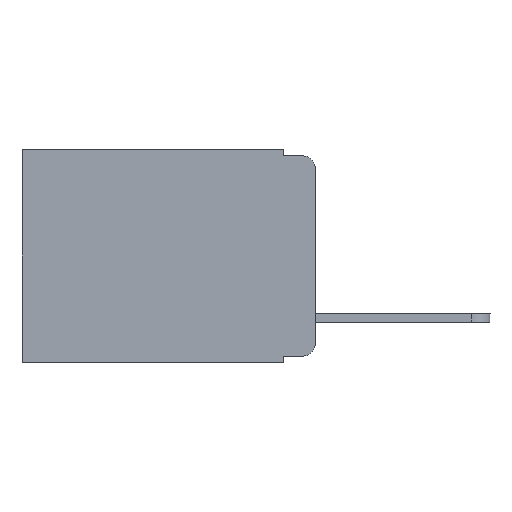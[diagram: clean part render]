
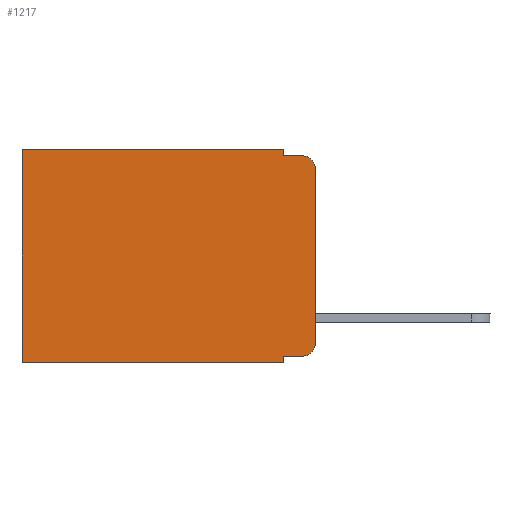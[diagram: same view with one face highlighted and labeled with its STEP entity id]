
A CAD part, left-side view. The second image highlights one B-rep face of the part: STEP entity #1217.
In plain terms, the highlighted planar face has unit normal (-1, 0, 0).
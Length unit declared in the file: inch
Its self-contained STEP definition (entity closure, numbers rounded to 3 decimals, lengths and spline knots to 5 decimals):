
#70 = LINE ( 'NONE', #7449, #6795 ) ;
#128 = DIRECTION ( 'NONE',  ( 0., -1., 0. ) ) ;
#259 = DIRECTION ( 'NONE',  ( 1., 0., 0. ) ) ;
#379 = LINE ( 'NONE', #4510, #958 ) ;
#500 = AXIS2_PLACEMENT_3D ( 'NONE', #8496, #259, #9436 ) ;
#527 = VECTOR ( 'NONE', #7770, 39.37008 ) ;
#958 = VECTOR ( 'NONE', #9495, 39.37008 ) ;
#1052 = ORIENTED_EDGE ( 'NONE', *, *, #6615, .T. ) ;
#1217 = ADVANCED_FACE ( 'NONE', ( #2091 ), #8603, .F. ) ;
#1247 = VERTEX_POINT ( 'NONE', #5398 ) ;
#1277 = EDGE_CURVE ( 'NONE', #10325, #5778, #3672, .T. ) ;
#1476 = EDGE_CURVE ( 'NONE', #10198, #7300, #3447, .T. ) ;
#2063 = EDGE_LOOP ( 'NONE', ( #9683, #9209, #2911, #2968, #3103, #5845, #3610, #7647, #1052, #7793 ) ) ;
#2086 = DIRECTION ( 'NONE',  ( 0., 0., -1. ) ) ;
#2091 = FACE_OUTER_BOUND ( 'NONE', #2063, .T. ) ;
#2202 = EDGE_CURVE ( 'NONE', #8750, #1247, #2500, .T. ) ;
#2421 = VECTOR ( 'NONE', #4393, 39.37008 ) ;
#2500 = CIRCLE ( 'NONE', #3886, 0.02 ) ;
#2911 = ORIENTED_EDGE ( 'NONE', *, *, #9700, .F. ) ;
#2965 = VERTEX_POINT ( 'NONE', #10240 ) ;
#2968 = ORIENTED_EDGE ( 'NONE', *, *, #1476, .F. ) ;
#3103 = ORIENTED_EDGE ( 'NONE', *, *, #5507, .T. ) ;
#3174 = EDGE_CURVE ( 'NONE', #8750, #7271, #70, .T. ) ;
#3294 = DIRECTION ( 'NONE',  ( 0., 0., -1. ) ) ;
#3352 = CARTESIAN_POINT ( 'NONE',  ( 0.298, 0.051, -0.343 ) ) ;
#3365 = VERTEX_POINT ( 'NONE', #7817 ) ;
#3447 = LINE ( 'NONE', #4275, #4166 ) ;
#3610 = ORIENTED_EDGE ( 'NONE', *, *, #1277, .F. ) ;
#3672 = LINE ( 'NONE', #6968, #2421 ) ;
#3679 = VECTOR ( 'NONE', #5118, 39.37008 ) ;
#3886 = AXIS2_PLACEMENT_3D ( 'NONE', #5590, #7159, #8031 ) ;
#3921 = CARTESIAN_POINT ( 'NONE',  ( 0.298, 0.051, -0.01 ) ) ;
#4166 = VECTOR ( 'NONE', #3294, 39.37008 ) ;
#4275 = CARTESIAN_POINT ( 'NONE',  ( 0.298, 0.051, 0. ) ) ;
#4365 = CARTESIAN_POINT ( 'NONE',  ( 0.298, 0.051, 0. ) ) ;
#4393 = DIRECTION ( 'NONE',  ( 0., 1., 0. ) ) ;
#4510 = CARTESIAN_POINT ( 'NONE',  ( 0.298, 0.051, -0.01 ) ) ;
#4614 = VERTEX_POINT ( 'NONE', #10211 ) ;
#5053 = EDGE_CURVE ( 'NONE', #4614, #7271, #9232, .T. ) ;
#5118 = DIRECTION ( 'NONE',  ( 0., 0., -1. ) ) ;
#5224 = LINE ( 'NONE', #6079, #527 ) ;
#5264 = EDGE_CURVE ( 'NONE', #2965, #5778, #7232, .T. ) ;
#5293 = CARTESIAN_POINT ( 'NONE',  ( 0.298, 0., -0.03 ) ) ;
#5398 = CARTESIAN_POINT ( 'NONE',  ( 0.298, 0.02, -0.01 ) ) ;
#5404 = AXIS2_PLACEMENT_3D ( 'NONE', #6912, #7785, #8599 ) ;
#5507 = EDGE_CURVE ( 'NONE', #10198, #2965, #5224, .T. ) ;
#5564 = CARTESIAN_POINT ( 'NONE',  ( 0.298, 0.051, 0. ) ) ;
#5590 = CARTESIAN_POINT ( 'NONE',  ( 0.298, 0.02, -0.03 ) ) ;
#5664 = CARTESIAN_POINT ( 'NONE',  ( 0.298, 0.051, -0.333 ) ) ;
#5778 = VERTEX_POINT ( 'NONE', #9292 ) ;
#5845 = ORIENTED_EDGE ( 'NONE', *, *, #5264, .T. ) ;
#6079 = CARTESIAN_POINT ( 'NONE',  ( 0.298, 0., 0. ) ) ;
#6615 = EDGE_CURVE ( 'NONE', #3365, #4614, #6744, .T. ) ;
#6744 = LINE ( 'NONE', #5664, #9224 ) ;
#6795 = VECTOR ( 'NONE', #7395, 39.37008 ) ;
#6912 = CARTESIAN_POINT ( 'NONE',  ( 0.298, 0.02, -0.313 ) ) ;
#6968 = CARTESIAN_POINT ( 'NONE',  ( 0.298, 0., -0.343 ) ) ;
#7047 = CARTESIAN_POINT ( 'NONE',  ( 0.298, 0., -0.313 ) ) ;
#7138 = EDGE_CURVE ( 'NONE', #3365, #10325, #10061, .T. ) ;
#7159 = DIRECTION ( 'NONE',  ( -1., 0., 0. ) ) ;
#7232 = LINE ( 'NONE', #10569, #9711 ) ;
#7271 = VERTEX_POINT ( 'NONE', #7047 ) ;
#7300 = VERTEX_POINT ( 'NONE', #3921 ) ;
#7395 = DIRECTION ( 'NONE',  ( 0., 0., -1. ) ) ;
#7449 = CARTESIAN_POINT ( 'NONE',  ( 0.298, 0., 0. ) ) ;
#7647 = ORIENTED_EDGE ( 'NONE', *, *, #7138, .F. ) ;
#7770 = DIRECTION ( 'NONE',  ( 0., 1., 0. ) ) ;
#7785 = DIRECTION ( 'NONE',  ( -1., 0., 0. ) ) ;
#7793 = ORIENTED_EDGE ( 'NONE', *, *, #5053, .T. ) ;
#7817 = CARTESIAN_POINT ( 'NONE',  ( 0.298, 0.051, -0.333 ) ) ;
#8031 = DIRECTION ( 'NONE',  ( 0., 0., -1. ) ) ;
#8496 = CARTESIAN_POINT ( 'NONE',  ( 0.298, 0., 0. ) ) ;
#8599 = DIRECTION ( 'NONE',  ( 0., 0., -1. ) ) ;
#8603 = PLANE ( 'NONE',  #500 ) ;
#8750 = VERTEX_POINT ( 'NONE', #5293 ) ;
#9209 = ORIENTED_EDGE ( 'NONE', *, *, #2202, .T. ) ;
#9224 = VECTOR ( 'NONE', #128, 39.37008 ) ;
#9232 = CIRCLE ( 'NONE', #5404, 0.02 ) ;
#9292 = CARTESIAN_POINT ( 'NONE',  ( 0.298, 0.473, -0.343 ) ) ;
#9436 = DIRECTION ( 'NONE',  ( 0., 0., -1. ) ) ;
#9495 = DIRECTION ( 'NONE',  ( 0., -1., 0. ) ) ;
#9683 = ORIENTED_EDGE ( 'NONE', *, *, #3174, .F. ) ;
#9700 = EDGE_CURVE ( 'NONE', #7300, #1247, #379, .T. ) ;
#9711 = VECTOR ( 'NONE', #2086, 39.37008 ) ;
#10061 = LINE ( 'NONE', #4365, #3679 ) ;
#10198 = VERTEX_POINT ( 'NONE', #5564 ) ;
#10211 = CARTESIAN_POINT ( 'NONE',  ( 0.298, 0.02, -0.333 ) ) ;
#10240 = CARTESIAN_POINT ( 'NONE',  ( 0.298, 0.473, 0. ) ) ;
#10325 = VERTEX_POINT ( 'NONE', #3352 ) ;
#10569 = CARTESIAN_POINT ( 'NONE',  ( 0.298, 0.473, 0. ) ) ;
